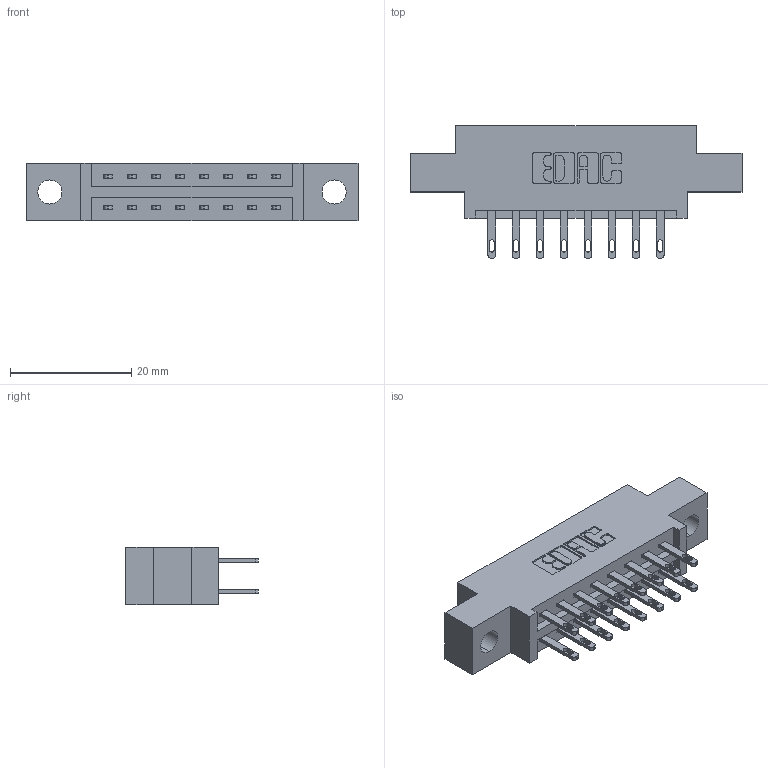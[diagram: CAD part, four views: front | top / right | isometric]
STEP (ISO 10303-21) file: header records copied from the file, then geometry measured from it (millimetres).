
FILE_DESCRIPTION (( 'STEP AP203' ), '1' );
FILE_NAME ('887-016-500-804.STEP', '2020-09-20T17:22:13', ( '' ), ( '' ), 'SwSTEP 2.0', 'SolidWorks 2020', '' );
FILE_SCHEMA (( 'CONFIG_CONTROL_DESIGN' ));
Length unit declared in the file: inch
Products named in the file (3): 887-016-500-804; 837 Part_0.170 Offset - 0.156 Dia-TH; 345-292-001_345-293-100
Assembly tree (17 placements, depth 2):
  887-016-500-804
    837 Part_0.170 Offset - 0.156 Dia-TH
    345-292-001_345-293-100  x16
Bounding box: 54.71 x 21.85 x 9.4 mm (x, y, z)
Volume: 5156.9 mm3; surface area: 5582.4 mm2
Topology: 17 solids, 17 shells, 918 faces, 2771 edges, 1846 vertices
Faces by surface type: plane 586, cylinder 332
Entity records: 10665 total; most frequent: CARTESIAN_POINT 1826, ORIENTED_EDGE 1762, DIRECTION 1617, EDGE_CURVE 881, VECTOR 749, LINE 749, VERTEX_POINT 586, AXIS2_PLACEMENT_3D 434
